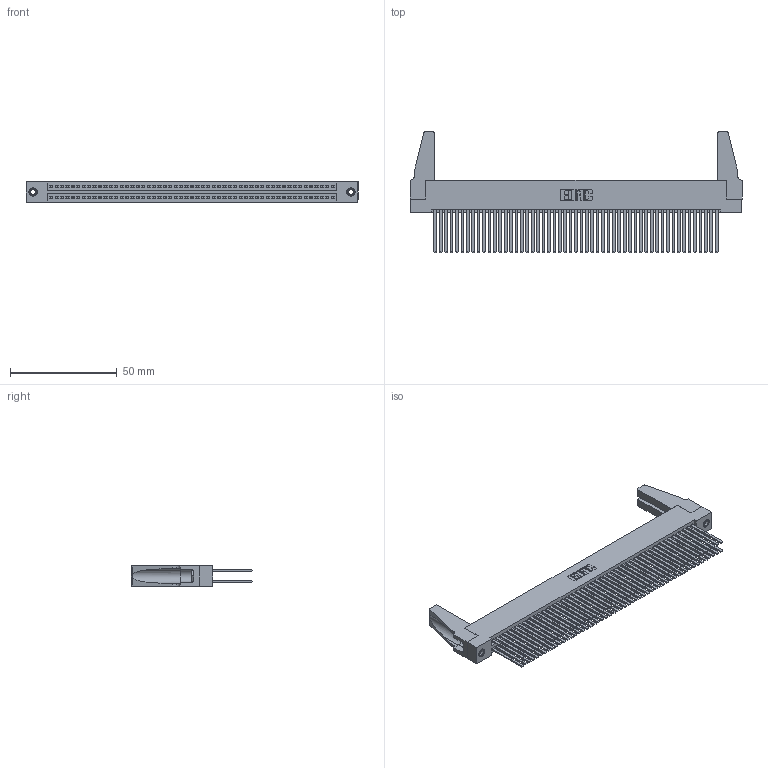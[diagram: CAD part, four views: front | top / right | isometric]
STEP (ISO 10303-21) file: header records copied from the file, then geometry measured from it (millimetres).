
FILE_DESCRIPTION (( 'STEP AP203' ), '1' );
FILE_NAME ('395-106-544-288.STEP', '2019-10-27T05:38:43', ( '' ), ( '' ), 'SwSTEP 2.0', 'SolidWorks 2016', '' );
FILE_SCHEMA (( 'CONFIG_CONTROL_DESIGN' ));
Length unit declared in the file: inch
Products named in the file (5): 345-220-078_345-220-088; 395-106-544-288; 345 Part_Flush Mounting Lugs - 0.156 Dia-TH; 345-292-001_345-293-144; 345-250-001_345-250-001-102
Assembly tree (111 placements, depth 2):
  395-106-544-288
    345 Part_Flush Mounting Lugs - 0.156 Dia-TH
    345-292-001_345-293-144  x106
    345-250-001_345-250-001-102  x2
    345-220-078_345-220-088  x2
Bounding box: 155.85 x 56.82 x 9.4 mm (x, y, z)
Volume: 19980.3 mm3; surface area: 32416.9 mm2
Topology: 111 solids, 111 shells, 4914 faces, 14541 edges, 9542 vertices
Faces by surface type: plane 3226, cylinder 1672, cone 12, torus 4
Entity records: 42068 total; most frequent: CARTESIAN_POINT 7034, ORIENTED_EDGE 6928, DIRECTION 6192, EDGE_CURVE 3464, LINE 3082, VECTOR 3082, VERTEX_POINT 2302, AXIS2_PLACEMENT_3D 1555
